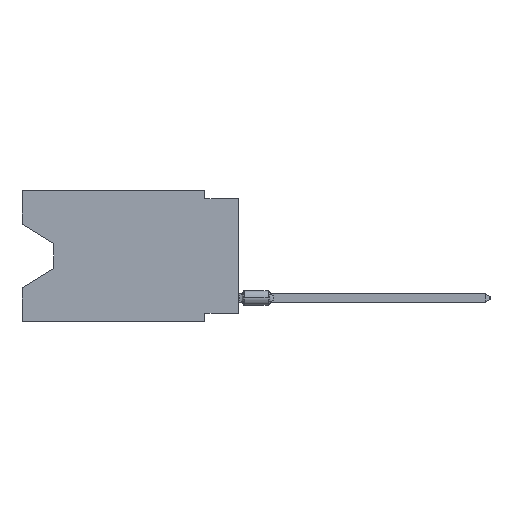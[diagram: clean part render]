
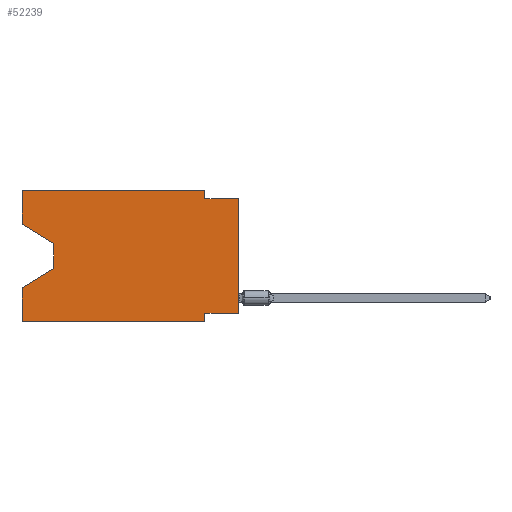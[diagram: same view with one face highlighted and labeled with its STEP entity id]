
A CAD part, left-side view. The second image highlights one B-rep face of the part: STEP entity #52239.
In plain terms, the highlighted planar face has unit normal (-1, 0, 0).
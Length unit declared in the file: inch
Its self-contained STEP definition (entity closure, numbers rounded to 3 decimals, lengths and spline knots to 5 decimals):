
#682 = DIRECTION ( 'NONE',  ( 0., 0., -1. ) ) ;
#755 = DIRECTION ( 'NONE',  ( 0., -1., 0. ) ) ;
#2331 = ORIENTED_EDGE ( 'NONE', *, *, #85315, .T. ) ;
#2828 = VECTOR ( 'NONE', #60042, 39.37008 ) ;
#4629 = FACE_OUTER_BOUND ( 'NONE', #66569, .T. ) ;
#4743 = VERTEX_POINT ( 'NONE', #18457 ) ;
#6638 = VERTEX_POINT ( 'NONE', #6889 ) ;
#6889 = CARTESIAN_POINT ( 'NONE',  ( 0., 0.55, -0.158 ) ) ;
#7530 = VERTEX_POINT ( 'NONE', #28707 ) ;
#8016 = CARTESIAN_POINT ( 'NONE',  ( 0., 0.645, 0. ) ) ;
#8042 = EDGE_CURVE ( 'NONE', #77309, #12510, #48434, .T. ) ;
#8634 = VECTOR ( 'NONE', #15646, 39.37008 ) ;
#8982 = LINE ( 'NONE', #14588, #42472 ) ;
#9641 = ORIENTED_EDGE ( 'NONE', *, *, #39682, .F. ) ;
#9643 = CARTESIAN_POINT ( 'NONE',  ( 0., 0., -0.365 ) ) ;
#10048 = LINE ( 'NONE', #24247, #72721 ) ;
#10607 = VERTEX_POINT ( 'NONE', #9643 ) ;
#10766 = EDGE_CURVE ( 'NONE', #10607, #7530, #27678, .T. ) ;
#10811 = VERTEX_POINT ( 'NONE', #74299 ) ;
#12510 = VERTEX_POINT ( 'NONE', #35349 ) ;
#12556 = DIRECTION ( 'NONE',  ( 0., 0., -1. ) ) ;
#14588 = CARTESIAN_POINT ( 'NONE',  ( 0., 0.645, -0.39 ) ) ;
#15646 = DIRECTION ( 'NONE',  ( 0., 0., -1. ) ) ;
#15729 = EDGE_CURVE ( 'NONE', #78671, #16037, #20973, .T. ) ;
#16037 = VERTEX_POINT ( 'NONE', #53666 ) ;
#16945 = DIRECTION ( 'NONE',  ( 0., -1., 0. ) ) ;
#18010 = DIRECTION ( 'NONE',  ( 1., 0., 0. ) ) ;
#18457 = CARTESIAN_POINT ( 'NONE',  ( 0., 0.1, -0.025 ) ) ;
#19713 = DIRECTION ( 'NONE',  ( 0., 0.855, -0.519 ) ) ;
#20973 = LINE ( 'NONE', #8016, #33488 ) ;
#23180 = EDGE_CURVE ( 'NONE', #16037, #35182, #10048, .T. ) ;
#24247 = CARTESIAN_POINT ( 'NONE',  ( 0., 0.645, 0. ) ) ;
#24372 = LINE ( 'NONE', #71824, #37118 ) ;
#26483 = VECTOR ( 'NONE', #36347, 39.37008 ) ;
#27134 = EDGE_CURVE ( 'NONE', #46497, #12510, #8982, .T. ) ;
#27579 = VECTOR ( 'NONE', #12556, 39.37008 ) ;
#27624 = VECTOR ( 'NONE', #49315, 39.37008 ) ;
#27678 = LINE ( 'NONE', #34145, #2828 ) ;
#28042 = ORIENTED_EDGE ( 'NONE', *, *, #51566, .F. ) ;
#28707 = CARTESIAN_POINT ( 'NONE',  ( 0., 0., -0.025 ) ) ;
#29553 = VECTOR ( 'NONE', #66100, 39.37008 ) ;
#30965 = CARTESIAN_POINT ( 'NONE',  ( 0., 0.645, 0. ) ) ;
#31385 = PLANE ( 'NONE',  #39060 ) ;
#32818 = ORIENTED_EDGE ( 'NONE', *, *, #8042, .F. ) ;
#33488 = VECTOR ( 'NONE', #53341, 39.37008 ) ;
#34145 = CARTESIAN_POINT ( 'NONE',  ( 0., 0., 0. ) ) ;
#34207 = CARTESIAN_POINT ( 'NONE',  ( 0., 0.1, 0. ) ) ;
#35182 = VERTEX_POINT ( 'NONE', #53638 ) ;
#35349 = CARTESIAN_POINT ( 'NONE',  ( 0., 0.1, -0.39 ) ) ;
#36347 = DIRECTION ( 'NONE',  ( 0., 0., 1. ) ) ;
#37118 = VECTOR ( 'NONE', #45492, 39.37008 ) ;
#39060 = AXIS2_PLACEMENT_3D ( 'NONE', #30965, #18010, #682 ) ;
#39544 = EDGE_CURVE ( 'NONE', #35182, #4743, #48868, .T. ) ;
#39682 = EDGE_CURVE ( 'NONE', #46497, #42706, #43652, .T. ) ;
#39757 = CARTESIAN_POINT ( 'NONE',  ( 0., 0., -0.025 ) ) ;
#40210 = ORIENTED_EDGE ( 'NONE', *, *, #23180, .F. ) ;
#40723 = ORIENTED_EDGE ( 'NONE', *, *, #39544, .F. ) ;
#42472 = VECTOR ( 'NONE', #755, 39.37008 ) ;
#42706 = VERTEX_POINT ( 'NONE', #48860 ) ;
#42822 = CARTESIAN_POINT ( 'NONE',  ( 0., 0.645, 0. ) ) ;
#43652 = LINE ( 'NONE', #42822, #26483 ) ;
#45492 = DIRECTION ( 'NONE',  ( 0., 1., 0. ) ) ;
#46497 = VERTEX_POINT ( 'NONE', #63426 ) ;
#48382 = LINE ( 'NONE', #39757, #29553 ) ;
#48434 = LINE ( 'NONE', #75202, #8634 ) ;
#48860 = CARTESIAN_POINT ( 'NONE',  ( 0., 0.645, -0.28975 ) ) ;
#48868 = LINE ( 'NONE', #34207, #70590 ) ;
#49315 = DIRECTION ( 'NONE',  ( 0., -0.855, -0.519 ) ) ;
#51399 = CARTESIAN_POINT ( 'NONE',  ( 0., 0.55, -0.158 ) ) ;
#51566 = EDGE_CURVE ( 'NONE', #10607, #77309, #24372, .T. ) ;
#52239 = ADVANCED_FACE ( 'NONE', ( #4629 ), #31385, .F. ) ;
#53341 = DIRECTION ( 'NONE',  ( 0., 0., 1. ) ) ;
#53638 = CARTESIAN_POINT ( 'NONE',  ( 0., 0.1, 0. ) ) ;
#53666 = CARTESIAN_POINT ( 'NONE',  ( 0., 0.645, 0. ) ) ;
#54513 = CARTESIAN_POINT ( 'NONE',  ( 0., 0.645, -0.10025 ) ) ;
#54525 = CARTESIAN_POINT ( 'NONE',  ( 0., 0.1, -0.365 ) ) ;
#55349 = DIRECTION ( 'NONE',  ( 0., 0., -1. ) ) ;
#60042 = DIRECTION ( 'NONE',  ( 0., 0., 1. ) ) ;
#60323 = ORIENTED_EDGE ( 'NONE', *, *, #15729, .F. ) ;
#61076 = ORIENTED_EDGE ( 'NONE', *, *, #67927, .T. ) ;
#61424 = LINE ( 'NONE', #54513, #27624 ) ;
#61897 = EDGE_CURVE ( 'NONE', #6638, #10811, #71675, .T. ) ;
#63258 = VECTOR ( 'NONE', #19713, 39.37008 ) ;
#63426 = CARTESIAN_POINT ( 'NONE',  ( 0., 0.645, -0.39 ) ) ;
#65903 = CARTESIAN_POINT ( 'NONE',  ( 0., 0.55, -0.232 ) ) ;
#66100 = DIRECTION ( 'NONE',  ( 0., -1., 0. ) ) ;
#66569 = EDGE_LOOP ( 'NONE', ( #61076, #83388, #2331, #9641, #81934, #32818, #28042, #72673, #76798, #40723, #40210, #60323 ) ) ;
#67927 = EDGE_CURVE ( 'NONE', #78671, #6638, #61424, .T. ) ;
#70590 = VECTOR ( 'NONE', #55349, 39.37008 ) ;
#71675 = LINE ( 'NONE', #51399, #27579 ) ;
#71824 = CARTESIAN_POINT ( 'NONE',  ( 0., 0., -0.365 ) ) ;
#72673 = ORIENTED_EDGE ( 'NONE', *, *, #10766, .T. ) ;
#72721 = VECTOR ( 'NONE', #16945, 39.37008 ) ;
#74299 = CARTESIAN_POINT ( 'NONE',  ( 0., 0.55, -0.232 ) ) ;
#75202 = CARTESIAN_POINT ( 'NONE',  ( 0., 0.1, -0.39 ) ) ;
#76798 = ORIENTED_EDGE ( 'NONE', *, *, #77801, .F. ) ;
#77119 = CARTESIAN_POINT ( 'NONE',  ( 0., 0.645, -0.10025 ) ) ;
#77309 = VERTEX_POINT ( 'NONE', #54525 ) ;
#77801 = EDGE_CURVE ( 'NONE', #4743, #7530, #48382, .T. ) ;
#78671 = VERTEX_POINT ( 'NONE', #77119 ) ;
#79294 = LINE ( 'NONE', #65903, #63258 ) ;
#81934 = ORIENTED_EDGE ( 'NONE', *, *, #27134, .T. ) ;
#83388 = ORIENTED_EDGE ( 'NONE', *, *, #61897, .T. ) ;
#85315 = EDGE_CURVE ( 'NONE', #10811, #42706, #79294, .T. ) ;
